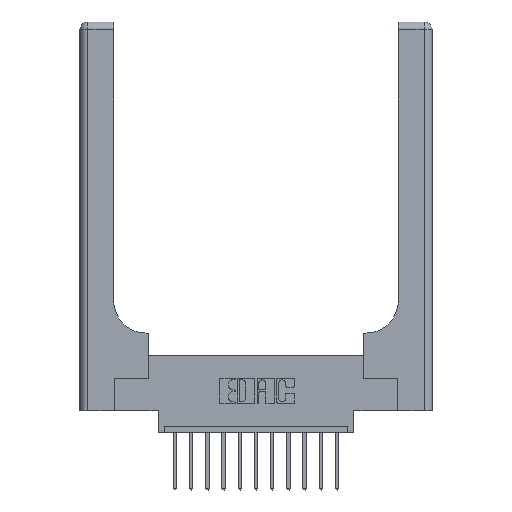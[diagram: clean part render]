
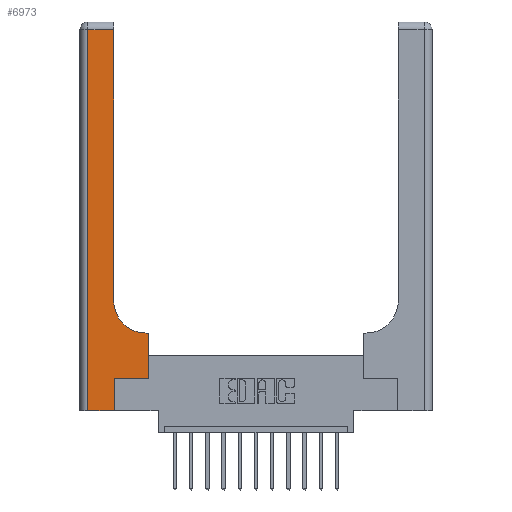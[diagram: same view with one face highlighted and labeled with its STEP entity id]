
A CAD part, top view. The second image highlights one B-rep face of the part: STEP entity #6973.
In plain terms, the highlighted planar face has unit normal (0, 0, 1).
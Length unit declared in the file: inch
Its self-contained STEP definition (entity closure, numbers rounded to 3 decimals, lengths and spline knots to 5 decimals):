
#129 = DIRECTION ( 'NONE',  ( 0., 1., 0. ) ) ;
#265 = EDGE_CURVE ( 'NONE', #4282, #13217, #15670, .T. ) ;
#629 = VECTOR ( 'NONE', #10843, 39.37008 ) ;
#1316 = CARTESIAN_POINT ( 'NONE',  ( 0.06, 0., 0.37 ) ) ;
#1927 = VECTOR ( 'NONE', #129, 39.37008 ) ;
#2082 = VERTEX_POINT ( 'NONE', #8143 ) ;
#2641 = VERTEX_POINT ( 'NONE', #4342 ) ;
#2665 = ORIENTED_EDGE ( 'NONE', *, *, #265, .T. ) ;
#2836 = ORIENTED_EDGE ( 'NONE', *, *, #5298, .T. ) ;
#2850 = CARTESIAN_POINT ( 'NONE',  ( 0.528, 0.25, 0.37 ) ) ;
#3481 = FACE_OUTER_BOUND ( 'NONE', #12237, .T. ) ;
#3645 = AXIS2_PLACEMENT_3D ( 'NONE', #11182, #7182, #11260 ) ;
#3909 = VERTEX_POINT ( 'NONE', #1316 ) ;
#4195 = VERTEX_POINT ( 'NONE', #15303 ) ;
#4282 = VERTEX_POINT ( 'NONE', #8994 ) ;
#4342 = CARTESIAN_POINT ( 'NONE',  ( 0.26, 0.85, 0.37 ) ) ;
#4376 = CARTESIAN_POINT ( 'NONE',  ( 0.26, 0.6, 0.37 ) ) ;
#4624 = DIRECTION ( 'NONE',  ( 1., 0., 0. ) ) ;
#4674 = LINE ( 'NONE', #8544, #4886 ) ;
#4732 = VECTOR ( 'NONE', #14388, 39.37008 ) ;
#4886 = VECTOR ( 'NONE', #9815, 39.37008 ) ;
#5128 = EDGE_CURVE ( 'NONE', #5932, #4195, #6733, .T. ) ;
#5298 = EDGE_CURVE ( 'NONE', #2082, #2641, #14709, .T. ) ;
#5696 = CARTESIAN_POINT ( 'NONE',  ( 0.265, 0., 0.37 ) ) ;
#5768 = LINE ( 'NONE', #8199, #629 ) ;
#5823 = CARTESIAN_POINT ( 'NONE',  ( 0.528, 0.6, 0.37 ) ) ;
#5882 = DIRECTION ( 'NONE',  ( 0., 0., -1. ) ) ;
#5932 = VERTEX_POINT ( 'NONE', #10164 ) ;
#6107 = DIRECTION ( 'NONE',  ( 1., 0., 0. ) ) ;
#6110 = EDGE_CURVE ( 'NONE', #2641, #5932, #5768, .T. ) ;
#6416 = EDGE_CURVE ( 'NONE', #13217, #2082, #14889, .T. ) ;
#6733 = LINE ( 'NONE', #14466, #4732 ) ;
#6973 = ADVANCED_FACE ( 'NONE', ( #3481 ), #16602, .F. ) ;
#7182 = DIRECTION ( 'NONE',  ( 0., 0., -1. ) ) ;
#7291 = CARTESIAN_POINT ( 'NONE',  ( 0.265, 0.25, 0.37 ) ) ;
#7875 = VERTEX_POINT ( 'NONE', #7291 ) ;
#7941 = VECTOR ( 'NONE', #9765, 39.37008 ) ;
#8054 = VECTOR ( 'NONE', #6107, 39.37008 ) ;
#8143 = CARTESIAN_POINT ( 'NONE',  ( 0.51, 0.6, 0.37 ) ) ;
#8199 = CARTESIAN_POINT ( 'NONE',  ( 0.26, 3., 0.37 ) ) ;
#8544 = CARTESIAN_POINT ( 'NONE',  ( 0.265, 0., 0.37 ) ) ;
#8825 = ORIENTED_EDGE ( 'NONE', *, *, #6110, .T. ) ;
#8902 = CARTESIAN_POINT ( 'NONE',  ( 0.06, 3., 0.37 ) ) ;
#8994 = CARTESIAN_POINT ( 'NONE',  ( 0.528, 0.25, 0.37 ) ) ;
#9251 = ORIENTED_EDGE ( 'NONE', *, *, #5128, .T. ) ;
#9515 = CARTESIAN_POINT ( 'NONE',  ( 0.51, 0.85, 0.37 ) ) ;
#9584 = ORIENTED_EDGE ( 'NONE', *, *, #10365, .T. ) ;
#9765 = DIRECTION ( 'NONE',  ( -1., 0., 0. ) ) ;
#9777 = ORIENTED_EDGE ( 'NONE', *, *, #11553, .T. ) ;
#9815 = DIRECTION ( 'NONE',  ( 0., 1., 0. ) ) ;
#10001 = EDGE_CURVE ( 'NONE', #7875, #4282, #11757, .T. ) ;
#10164 = CARTESIAN_POINT ( 'NONE',  ( 0.26, 2.94, 0.37 ) ) ;
#10365 = EDGE_CURVE ( 'NONE', #4195, #3909, #11122, .T. ) ;
#10480 = CARTESIAN_POINT ( 'NONE',  ( 0.265, 0.25, 0.37 ) ) ;
#10843 = DIRECTION ( 'NONE',  ( 0., 1., 0. ) ) ;
#11122 = LINE ( 'NONE', #8902, #11829 ) ;
#11182 = CARTESIAN_POINT ( 'NONE',  ( 0., 3., 0.37 ) ) ;
#11187 = CARTESIAN_POINT ( 'NONE',  ( 0., 0., 0.37 ) ) ;
#11260 = DIRECTION ( 'NONE',  ( -1., 0., 0. ) ) ;
#11432 = VERTEX_POINT ( 'NONE', #5696 ) ;
#11553 = EDGE_CURVE ( 'NONE', #3909, #11432, #13731, .T. ) ;
#11558 = VECTOR ( 'NONE', #15681, 39.37008 ) ;
#11757 = LINE ( 'NONE', #10480, #11558 ) ;
#11829 = VECTOR ( 'NONE', #14097, 39.37008 ) ;
#12237 = EDGE_LOOP ( 'NONE', ( #8825, #9251, #9584, #9777, #13368, #12549, #2665, #15135, #2836 ) ) ;
#12549 = ORIENTED_EDGE ( 'NONE', *, *, #10001, .T. ) ;
#13217 = VERTEX_POINT ( 'NONE', #5823 ) ;
#13368 = ORIENTED_EDGE ( 'NONE', *, *, #15270, .T. ) ;
#13374 = AXIS2_PLACEMENT_3D ( 'NONE', #9515, #5882, #4624 ) ;
#13731 = LINE ( 'NONE', #11187, #8054 ) ;
#14097 = DIRECTION ( 'NONE',  ( 0., -1., 0. ) ) ;
#14388 = DIRECTION ( 'NONE',  ( -1., 0., 0. ) ) ;
#14466 = CARTESIAN_POINT ( 'NONE',  ( 0., 2.94, 0.37 ) ) ;
#14709 = CIRCLE ( 'NONE', #13374, 0.25 ) ;
#14889 = LINE ( 'NONE', #4376, #7941 ) ;
#15135 = ORIENTED_EDGE ( 'NONE', *, *, #6416, .T. ) ;
#15270 = EDGE_CURVE ( 'NONE', #11432, #7875, #4674, .T. ) ;
#15303 = CARTESIAN_POINT ( 'NONE',  ( 0.06, 2.94, 0.37 ) ) ;
#15670 = LINE ( 'NONE', #2850, #1927 ) ;
#15681 = DIRECTION ( 'NONE',  ( 1., 0., 0. ) ) ;
#16602 = PLANE ( 'NONE',  #3645 ) ;
